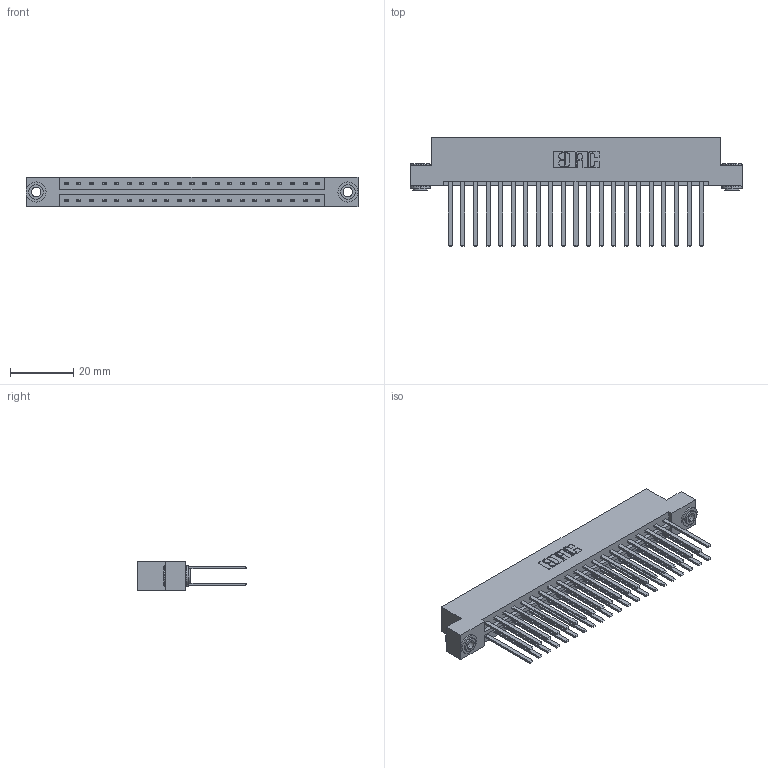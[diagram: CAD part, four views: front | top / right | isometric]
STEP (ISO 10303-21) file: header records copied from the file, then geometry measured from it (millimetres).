
FILE_DESCRIPTION (( 'STEP AP203' ), '1' );
FILE_NAME ('333-042-544-203.STEP', '2018-08-03T19:17:37', ( '' ), ( '' ), 'SwSTEP 2.0', 'SolidWorks 2016', '' );
FILE_SCHEMA (( 'CONFIG_CONTROL_DESIGN' ));
Length unit declared in the file: inch
Products named in the file (4): 333 Part_Flush - .156 Dia - TH; 345-292-001_345-293-144; 345-250-002_345-250-002-102; 333-042-544-203
Assembly tree (45 placements, depth 2):
  333-042-544-203
    333 Part_Flush - .156 Dia - TH
    345-292-001_345-293-144  x42
    345-250-002_345-250-002-102  x2
Bounding box: 104.75 x 34.3 x 9.4 mm (x, y, z)
Volume: 11106.1 mm3; surface area: 15021.1 mm2
Topology: 45 solids, 45 shells, 2084 faces, 6141 edges, 4034 vertices
Faces by surface type: plane 1424, cylinder 652, cone 8
Entity records: 16692 total; most frequent: CARTESIAN_POINT 2765, ORIENTED_EDGE 2694, DIRECTION 2429, EDGE_CURVE 1347, LINE 1199, VECTOR 1199, VERTEX_POINT 894, AXIS2_PLACEMENT_3D 615
